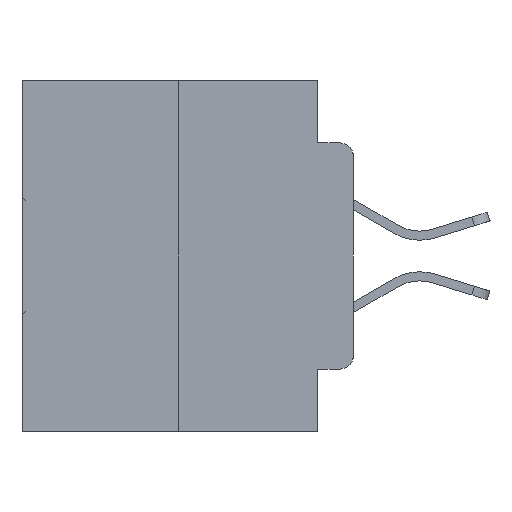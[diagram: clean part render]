
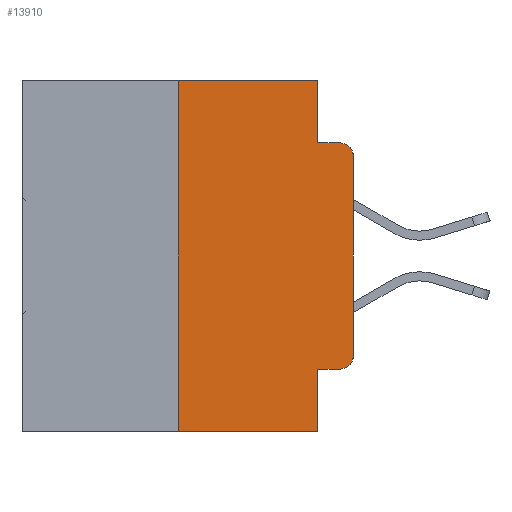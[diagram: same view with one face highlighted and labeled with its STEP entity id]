
A CAD part, left-side view. The second image highlights one B-rep face of the part: STEP entity #13910.
In plain terms, the highlighted planar face has unit normal (-1, 0, 0).
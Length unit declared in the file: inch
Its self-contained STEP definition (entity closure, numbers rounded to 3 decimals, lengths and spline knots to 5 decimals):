
#277 = ORIENTED_EDGE ( 'NONE', *, *, #3273, .T. ) ;
#918 = CARTESIAN_POINT ( 'NONE',  ( 0., 0.25, 0. ) ) ;
#970 = DIRECTION ( 'NONE',  ( -1., 0., 0. ) ) ;
#1089 = CARTESIAN_POINT ( 'NONE',  ( 0., 0.25, 0. ) ) ;
#1098 = ORIENTED_EDGE ( 'NONE', *, *, #9634, .F. ) ;
#1471 = CARTESIAN_POINT ( 'NONE',  ( 0., 0.02, -0.1085 ) ) ;
#1776 = VERTEX_POINT ( 'NONE', #26528 ) ;
#2844 = DIRECTION ( 'NONE',  ( 0., 0., -1. ) ) ;
#3273 = EDGE_CURVE ( 'NONE', #18722, #16980, #27747, .T. ) ;
#3785 = CARTESIAN_POINT ( 'NONE',  ( 0., 0.051, 0. ) ) ;
#3796 = DIRECTION ( 'NONE',  ( 0., 0., -1. ) ) ;
#3953 = DIRECTION ( 'NONE',  ( 0., 0., -1. ) ) ;
#5063 = CARTESIAN_POINT ( 'NONE',  ( 0., 0.051, 0. ) ) ;
#5247 = ORIENTED_EDGE ( 'NONE', *, *, #5700, .T. ) ;
#5414 = CARTESIAN_POINT ( 'NONE',  ( 0., 0.473, -0.5 ) ) ;
#5483 = DIRECTION ( 'NONE',  ( 0., 0., 1. ) ) ;
#5605 = LINE ( 'NONE', #5414, #31185 ) ;
#5700 = EDGE_CURVE ( 'NONE', #16980, #11868, #19783, .T. ) ;
#6307 = CARTESIAN_POINT ( 'NONE',  ( 0., 0.051, 0. ) ) ;
#6328 = EDGE_CURVE ( 'NONE', #1776, #21345, #17492, .T. ) ;
#6942 = EDGE_CURVE ( 'NONE', #1776, #12529, #5605, .T. ) ;
#7306 = CARTESIAN_POINT ( 'NONE',  ( 0., 0.02, -0.3915 ) ) ;
#7360 = DIRECTION ( 'NONE',  ( 0., -1., 0. ) ) ;
#7785 = CARTESIAN_POINT ( 'NONE',  ( 0., 0.051, -0.4115 ) ) ;
#8301 = CARTESIAN_POINT ( 'NONE',  ( 0., 0.051, -0.4115 ) ) ;
#8650 = LINE ( 'NONE', #28633, #27374 ) ;
#8698 = EDGE_LOOP ( 'NONE', ( #5247, #9598, #11801, #22413, #12560, #11139, #14962, #1098, #25430, #277 ) ) ;
#8946 = CIRCLE ( 'NONE', #12101, 0.02 ) ;
#9036 = EDGE_CURVE ( 'NONE', #11868, #13395, #8946, .T. ) ;
#9598 = ORIENTED_EDGE ( 'NONE', *, *, #9036, .T. ) ;
#9634 = EDGE_CURVE ( 'NONE', #28379, #12529, #27698, .T. ) ;
#10039 = VECTOR ( 'NONE', #24677, 39.37008 ) ;
#10183 = CARTESIAN_POINT ( 'NONE',  ( 0., 0.473, 0. ) ) ;
#11049 = CARTESIAN_POINT ( 'NONE',  ( 0., 0.02, -0.4115 ) ) ;
#11139 = ORIENTED_EDGE ( 'NONE', *, *, #6328, .F. ) ;
#11597 = AXIS2_PLACEMENT_3D ( 'NONE', #10183, #17502, #2844 ) ;
#11801 = ORIENTED_EDGE ( 'NONE', *, *, #20966, .F. ) ;
#11868 = VERTEX_POINT ( 'NONE', #20219 ) ;
#12101 = AXIS2_PLACEMENT_3D ( 'NONE', #1471, #18601, #3953 ) ;
#12529 = VERTEX_POINT ( 'NONE', #29654 ) ;
#12560 = ORIENTED_EDGE ( 'NONE', *, *, #14449, .F. ) ;
#12779 = LINE ( 'NONE', #14632, #24792 ) ;
#12902 = LINE ( 'NONE', #3785, #31176 ) ;
#13029 = VERTEX_POINT ( 'NONE', #5063 ) ;
#13395 = VERTEX_POINT ( 'NONE', #27949 ) ;
#13910 = ADVANCED_FACE ( 'NONE', ( #27047 ), #15092, .F. ) ;
#14236 = VECTOR ( 'NONE', #3796, 39.37008 ) ;
#14449 = EDGE_CURVE ( 'NONE', #21345, #13029, #12779, .T. ) ;
#14632 = CARTESIAN_POINT ( 'NONE',  ( 0., 0.473, 0. ) ) ;
#14962 = ORIENTED_EDGE ( 'NONE', *, *, #6942, .T. ) ;
#15092 = PLANE ( 'NONE',  #11597 ) ;
#16009 = VECTOR ( 'NONE', #26552, 39.37008 ) ;
#16444 = EDGE_CURVE ( 'NONE', #28379, #18722, #29157, .T. ) ;
#16980 = VERTEX_POINT ( 'NONE', #26352 ) ;
#17492 = LINE ( 'NONE', #918, #16009 ) ;
#17502 = DIRECTION ( 'NONE',  ( 1., 0., 0. ) ) ;
#18601 = DIRECTION ( 'NONE',  ( -1., 0., 0. ) ) ;
#18656 = CARTESIAN_POINT ( 'NONE',  ( 0., 0.051, -0.0885 ) ) ;
#18722 = VERTEX_POINT ( 'NONE', #11049 ) ;
#18778 = VERTEX_POINT ( 'NONE', #18656 ) ;
#19610 = AXIS2_PLACEMENT_3D ( 'NONE', #7306, #970, #25701 ) ;
#19783 = LINE ( 'NONE', #31023, #26113 ) ;
#20219 = CARTESIAN_POINT ( 'NONE',  ( 0., 0., -0.1085 ) ) ;
#20966 = EDGE_CURVE ( 'NONE', #18778, #13395, #8650, .T. ) ;
#21345 = VERTEX_POINT ( 'NONE', #1089 ) ;
#22413 = ORIENTED_EDGE ( 'NONE', *, *, #27345, .F. ) ;
#23855 = DIRECTION ( 'NONE',  ( 0., -1., 0. ) ) ;
#24677 = DIRECTION ( 'NONE',  ( 0., -1., 0. ) ) ;
#24792 = VECTOR ( 'NONE', #7360, 39.37008 ) ;
#25430 = ORIENTED_EDGE ( 'NONE', *, *, #16444, .T. ) ;
#25648 = DIRECTION ( 'NONE',  ( 0., 0., -1. ) ) ;
#25701 = DIRECTION ( 'NONE',  ( 0., 0., -1. ) ) ;
#26113 = VECTOR ( 'NONE', #5483, 39.37008 ) ;
#26352 = CARTESIAN_POINT ( 'NONE',  ( 0., 0., -0.3915 ) ) ;
#26528 = CARTESIAN_POINT ( 'NONE',  ( 0., 0.25, -0.5 ) ) ;
#26552 = DIRECTION ( 'NONE',  ( 0., 0., 1. ) ) ;
#26762 = DIRECTION ( 'NONE',  ( 0., -1., 0. ) ) ;
#27047 = FACE_OUTER_BOUND ( 'NONE', #8698, .T. ) ;
#27345 = EDGE_CURVE ( 'NONE', #13029, #18778, #12902, .T. ) ;
#27374 = VECTOR ( 'NONE', #23855, 39.37008 ) ;
#27698 = LINE ( 'NONE', #6307, #14236 ) ;
#27747 = CIRCLE ( 'NONE', #19610, 0.02 ) ;
#27949 = CARTESIAN_POINT ( 'NONE',  ( 0., 0.02, -0.0885 ) ) ;
#28379 = VERTEX_POINT ( 'NONE', #8301 ) ;
#28633 = CARTESIAN_POINT ( 'NONE',  ( 0., 0.051, -0.0885 ) ) ;
#29157 = LINE ( 'NONE', #7785, #10039 ) ;
#29654 = CARTESIAN_POINT ( 'NONE',  ( 0., 0.051, -0.5 ) ) ;
#31023 = CARTESIAN_POINT ( 'NONE',  ( 0., 0., 0. ) ) ;
#31176 = VECTOR ( 'NONE', #25648, 39.37008 ) ;
#31185 = VECTOR ( 'NONE', #26762, 39.37008 ) ;
